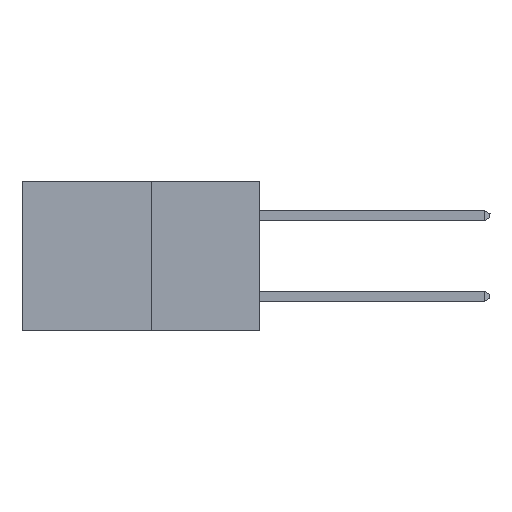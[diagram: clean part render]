
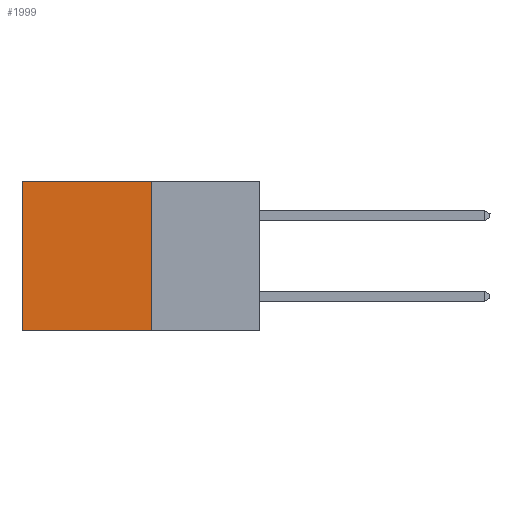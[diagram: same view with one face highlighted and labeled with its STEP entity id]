
A CAD part, left-side view. The second image highlights one B-rep face of the part: STEP entity #1999.
In plain terms, the highlighted planar face has unit normal (-1, 0, 0).
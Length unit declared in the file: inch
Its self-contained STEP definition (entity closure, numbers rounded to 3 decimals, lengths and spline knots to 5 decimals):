
#210 = VECTOR ( 'NONE', #8804, 39.37008 ) ;
#398 = EDGE_CURVE ( 'NONE', #2700, #5644, #6188, .T. ) ;
#979 = DIRECTION ( 'NONE',  ( 0., 1., 0. ) ) ;
#1314 = EDGE_CURVE ( 'NONE', #8951, #7536, #7975, .T. ) ;
#1668 = CARTESIAN_POINT ( 'NONE',  ( 0.277, 0.27, -0.37 ) ) ;
#1999 = ADVANCED_FACE ( 'NONE', ( #7381 ), #3695, .F. ) ;
#2697 = VECTOR ( 'NONE', #9894, 39.37008 ) ;
#2700 = VERTEX_POINT ( 'NONE', #10643 ) ;
#3022 = LINE ( 'NONE', #7043, #2697 ) ;
#3408 = ORIENTED_EDGE ( 'NONE', *, *, #1314, .T. ) ;
#3427 = VECTOR ( 'NONE', #10792, 39.37008 ) ;
#3482 = DIRECTION ( 'NONE',  ( 0., 0., -1. ) ) ;
#3485 = ORIENTED_EDGE ( 'NONE', *, *, #398, .F. ) ;
#3534 = DIRECTION ( 'NONE',  ( 1., 0., 0. ) ) ;
#3695 = PLANE ( 'NONE',  #5887 ) ;
#3699 = CARTESIAN_POINT ( 'NONE',  ( 0.277, 0.27, -0.37 ) ) ;
#4227 = ORIENTED_EDGE ( 'NONE', *, *, #5260, .F. ) ;
#5192 = VECTOR ( 'NONE', #979, 39.37008 ) ;
#5260 = EDGE_CURVE ( 'NONE', #5644, #7536, #12586, .T. ) ;
#5644 = VERTEX_POINT ( 'NONE', #1668 ) ;
#5698 = CARTESIAN_POINT ( 'NONE',  ( 0.277, 0.59, -0.37 ) ) ;
#5887 = AXIS2_PLACEMENT_3D ( 'NONE', #3699, #3534, #3482 ) ;
#6188 = LINE ( 'NONE', #9298, #3427 ) ;
#7043 = CARTESIAN_POINT ( 'NONE',  ( 0.277, 0.27, 0. ) ) ;
#7381 = FACE_OUTER_BOUND ( 'NONE', #11746, .T. ) ;
#7536 = VERTEX_POINT ( 'NONE', #5698 ) ;
#7975 = LINE ( 'NONE', #8310, #210 ) ;
#8104 = ORIENTED_EDGE ( 'NONE', *, *, #11380, .T. ) ;
#8310 = CARTESIAN_POINT ( 'NONE',  ( 0.277, 0.59, -0.37 ) ) ;
#8762 = CARTESIAN_POINT ( 'NONE',  ( 0.277, 0.59, 0. ) ) ;
#8804 = DIRECTION ( 'NONE',  ( 0., 0., -1. ) ) ;
#8951 = VERTEX_POINT ( 'NONE', #8762 ) ;
#9298 = CARTESIAN_POINT ( 'NONE',  ( 0.277, 0.27, -0.37 ) ) ;
#9894 = DIRECTION ( 'NONE',  ( 0., 1., 0. ) ) ;
#10643 = CARTESIAN_POINT ( 'NONE',  ( 0.277, 0.27, 0. ) ) ;
#10792 = DIRECTION ( 'NONE',  ( 0., 0., -1. ) ) ;
#11380 = EDGE_CURVE ( 'NONE', #2700, #8951, #3022, .T. ) ;
#11746 = EDGE_LOOP ( 'NONE', ( #3408, #4227, #3485, #8104 ) ) ;
#12586 = LINE ( 'NONE', #12626, #5192 ) ;
#12626 = CARTESIAN_POINT ( 'NONE',  ( 0.277, 0.27, -0.37 ) ) ;
